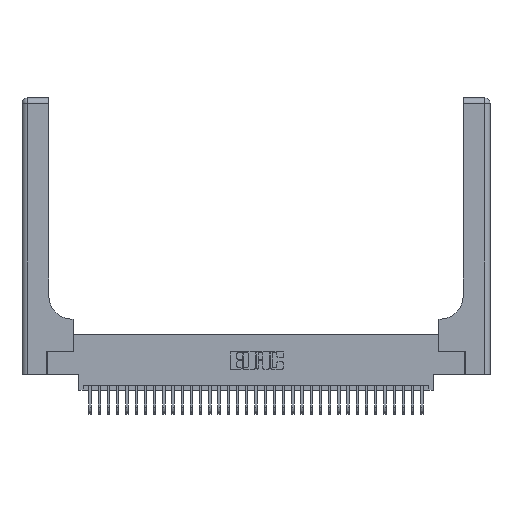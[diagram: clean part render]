
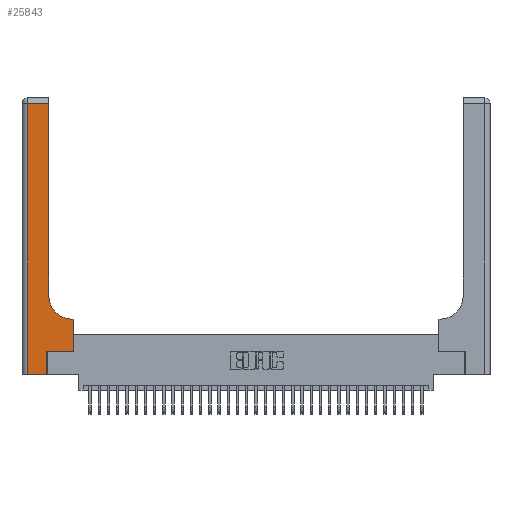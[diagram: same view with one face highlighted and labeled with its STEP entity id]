
A CAD part, top view. The second image highlights one B-rep face of the part: STEP entity #25843.
In plain terms, the highlighted planar face has unit normal (0, 0, 1).
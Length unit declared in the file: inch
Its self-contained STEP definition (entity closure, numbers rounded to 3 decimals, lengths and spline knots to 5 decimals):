
#341 = EDGE_CURVE ( 'NONE', #12256, #10644, #33066, .T. ) ;
#474 = DIRECTION ( 'NONE',  ( 1., 0., 0. ) ) ;
#715 = LINE ( 'NONE', #7004, #13006 ) ;
#874 = CARTESIAN_POINT ( 'NONE',  ( 0.269, 0., 0.37 ) ) ;
#1567 = CARTESIAN_POINT ( 'NONE',  ( 0., 3., 0.37 ) ) ;
#1909 = ORIENTED_EDGE ( 'NONE', *, *, #31182, .T. ) ;
#3208 = EDGE_CURVE ( 'NONE', #32788, #24657, #13572, .T. ) ;
#3956 = LINE ( 'NONE', #5842, #17886 ) ;
#4029 = FACE_OUTER_BOUND ( 'NONE', #16507, .T. ) ;
#4206 = PLANE ( 'NONE',  #10802 ) ;
#4454 = CIRCLE ( 'NONE', #24242, 0.25 ) ;
#4607 = CARTESIAN_POINT ( 'NONE',  ( 0.06, 3., 0.37 ) ) ;
#5353 = LINE ( 'NONE', #5988, #23782 ) ;
#5842 = CARTESIAN_POINT ( 'NONE',  ( 0.5585, 0.25, 0.37 ) ) ;
#5988 = CARTESIAN_POINT ( 'NONE',  ( 0., 0., 0.37 ) ) ;
#5995 = CARTESIAN_POINT ( 'NONE',  ( 0.5585, 0.25, 0.37 ) ) ;
#7004 = CARTESIAN_POINT ( 'NONE',  ( 0., 2.94, 0.37 ) ) ;
#8476 = DIRECTION ( 'NONE',  ( 0., 1., 0. ) ) ;
#8615 = DIRECTION ( 'NONE',  ( 1., 0., 0. ) ) ;
#8944 = EDGE_CURVE ( 'NONE', #31068, #9445, #14556, .T. ) ;
#9445 = VERTEX_POINT ( 'NONE', #14661 ) ;
#9468 = DIRECTION ( 'NONE',  ( -1., 0., 0. ) ) ;
#10274 = CARTESIAN_POINT ( 'NONE',  ( 0.2915, 3., 0.37 ) ) ;
#10644 = VERTEX_POINT ( 'NONE', #33006 ) ;
#10802 = AXIS2_PLACEMENT_3D ( 'NONE', #1567, #25164, #9468 ) ;
#11169 = CARTESIAN_POINT ( 'NONE',  ( 0.2915, 2.94, 0.37 ) ) ;
#11917 = CARTESIAN_POINT ( 'NONE',  ( 0.269, 0., 0.37 ) ) ;
#12256 = VERTEX_POINT ( 'NONE', #11917 ) ;
#12360 = EDGE_CURVE ( 'NONE', #29122, #32788, #4454, .T. ) ;
#12385 = CARTESIAN_POINT ( 'NONE',  ( 0.5415, 0.85, 0.37 ) ) ;
#12783 = VECTOR ( 'NONE', #26866, 39.37008 ) ;
#12852 = CARTESIAN_POINT ( 'NONE',  ( 0.2915, 0.85, 0.37 ) ) ;
#12895 = DIRECTION ( 'NONE',  ( 0., 1., 0. ) ) ;
#12951 = ORIENTED_EDGE ( 'NONE', *, *, #19423, .T. ) ;
#12989 = ORIENTED_EDGE ( 'NONE', *, *, #29592, .T. ) ;
#13006 = VECTOR ( 'NONE', #22791, 39.37008 ) ;
#13124 = LINE ( 'NONE', #18772, #32382 ) ;
#13200 = CARTESIAN_POINT ( 'NONE',  ( 0.06, 2.94, 0.37 ) ) ;
#13380 = ORIENTED_EDGE ( 'NONE', *, *, #341, .T. ) ;
#13572 = LINE ( 'NONE', #10274, #33660 ) ;
#14556 = LINE ( 'NONE', #4607, #28473 ) ;
#14661 = CARTESIAN_POINT ( 'NONE',  ( 0.06, 0., 0.37 ) ) ;
#15026 = DIRECTION ( 'NONE',  ( 1., 0., 0. ) ) ;
#16507 = EDGE_LOOP ( 'NONE', ( #32232, #12951, #28513, #17036, #13380, #1909, #30612, #12989, #29388 ) ) ;
#17036 = ORIENTED_EDGE ( 'NONE', *, *, #23360, .T. ) ;
#17886 = VECTOR ( 'NONE', #8476, 39.37008 ) ;
#18772 = CARTESIAN_POINT ( 'NONE',  ( 0.269, 0.25, 0.37 ) ) ;
#19423 = EDGE_CURVE ( 'NONE', #24657, #31068, #715, .T. ) ;
#19730 = EDGE_CURVE ( 'NONE', #28620, #28499, #3956, .T. ) ;
#21811 = DIRECTION ( 'NONE',  ( 0., 1., 0. ) ) ;
#22791 = DIRECTION ( 'NONE',  ( -1., 0., 0. ) ) ;
#23360 = EDGE_CURVE ( 'NONE', #9445, #12256, #5353, .T. ) ;
#23600 = CARTESIAN_POINT ( 'NONE',  ( 0.5415, 0.6, 0.37 ) ) ;
#23782 = VECTOR ( 'NONE', #8615, 39.37008 ) ;
#24242 = AXIS2_PLACEMENT_3D ( 'NONE', #12385, #30731, #15026 ) ;
#24256 = CARTESIAN_POINT ( 'NONE',  ( 0.2915, 0.6, 0.37 ) ) ;
#24657 = VERTEX_POINT ( 'NONE', #11169 ) ;
#25164 = DIRECTION ( 'NONE',  ( 0., 0., -1. ) ) ;
#25843 = ADVANCED_FACE ( 'NONE', ( #4029 ), #4206, .F. ) ;
#26070 = VECTOR ( 'NONE', #21811, 39.37008 ) ;
#26866 = DIRECTION ( 'NONE',  ( -1., 0., 0. ) ) ;
#28473 = VECTOR ( 'NONE', #33355, 39.37008 ) ;
#28499 = VERTEX_POINT ( 'NONE', #29020 ) ;
#28513 = ORIENTED_EDGE ( 'NONE', *, *, #8944, .T. ) ;
#28620 = VERTEX_POINT ( 'NONE', #5995 ) ;
#29020 = CARTESIAN_POINT ( 'NONE',  ( 0.5585, 0.6, 0.37 ) ) ;
#29122 = VERTEX_POINT ( 'NONE', #23600 ) ;
#29388 = ORIENTED_EDGE ( 'NONE', *, *, #12360, .T. ) ;
#29592 = EDGE_CURVE ( 'NONE', #28499, #29122, #33695, .T. ) ;
#30612 = ORIENTED_EDGE ( 'NONE', *, *, #19730, .T. ) ;
#30731 = DIRECTION ( 'NONE',  ( 0., 0., -1. ) ) ;
#31068 = VERTEX_POINT ( 'NONE', #13200 ) ;
#31182 = EDGE_CURVE ( 'NONE', #10644, #28620, #13124, .T. ) ;
#32232 = ORIENTED_EDGE ( 'NONE', *, *, #3208, .T. ) ;
#32382 = VECTOR ( 'NONE', #474, 39.37008 ) ;
#32788 = VERTEX_POINT ( 'NONE', #12852 ) ;
#33006 = CARTESIAN_POINT ( 'NONE',  ( 0.269, 0.25, 0.37 ) ) ;
#33066 = LINE ( 'NONE', #874, #26070 ) ;
#33355 = DIRECTION ( 'NONE',  ( 0., -1., 0. ) ) ;
#33660 = VECTOR ( 'NONE', #12895, 39.37008 ) ;
#33695 = LINE ( 'NONE', #24256, #12783 ) ;
